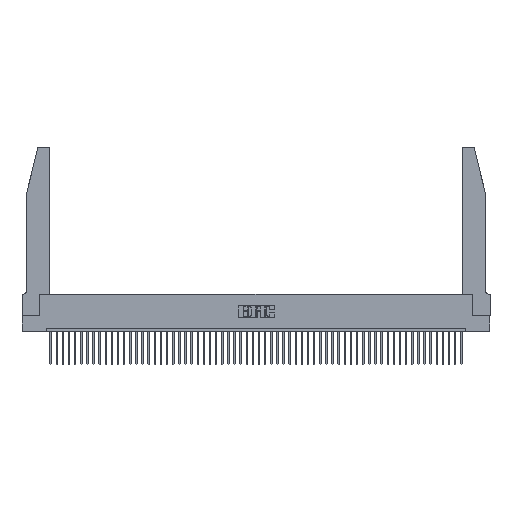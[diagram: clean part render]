
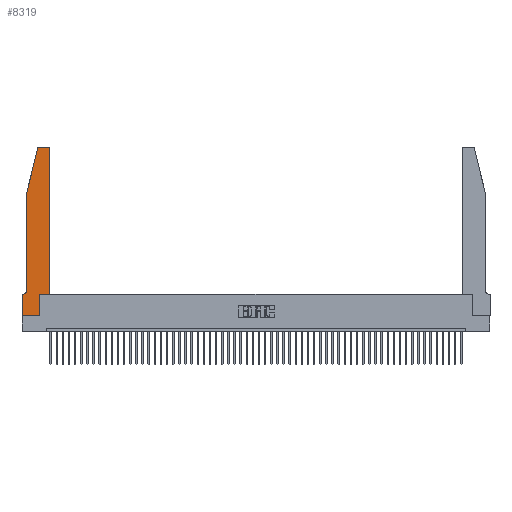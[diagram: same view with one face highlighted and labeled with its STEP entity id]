
A CAD part, top view. The second image highlights one B-rep face of the part: STEP entity #8319.
In plain terms, the highlighted planar face has unit normal (0, 0, 1).
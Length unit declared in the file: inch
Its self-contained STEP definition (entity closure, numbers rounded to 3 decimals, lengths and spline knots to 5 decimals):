
#94 = CARTESIAN_POINT ( 'NONE',  ( 0.2865, 0.35, 0.37 ) ) ;
#835 = EDGE_CURVE ( 'NONE', #48034, #19358, #24622, .T. ) ;
#1176 = DIRECTION ( 'NONE',  ( 0., -1., 0. ) ) ;
#1501 = EDGE_CURVE ( 'NONE', #41923, #16142, #8799, .T. ) ;
#1686 = EDGE_CURVE ( 'NONE', #50019, #41923, #30232, .T. ) ;
#1885 = CARTESIAN_POINT ( 'NONE',  ( 0., 0.35, 0.37 ) ) ;
#2378 = DIRECTION ( 'NONE',  ( 0., 1., 0. ) ) ;
#3093 = CARTESIAN_POINT ( 'NONE',  ( 0.0755, 2., 0.37 ) ) ;
#3177 = DIRECTION ( 'NONE',  ( 1., 0., 0. ) ) ;
#4430 = VECTOR ( 'NONE', #41938, 39.37008 ) ;
#5668 = CARTESIAN_POINT ( 'NONE',  ( 0.0755, 2., 0.37 ) ) ;
#5995 = EDGE_CURVE ( 'NONE', #42467, #19080, #8947, .T. ) ;
#6057 = DIRECTION ( 'NONE',  ( -0.239, -0.971, 0. ) ) ;
#6520 = CARTESIAN_POINT ( 'NONE',  ( 0.4505, 0.35, 0.37 ) ) ;
#6750 = EDGE_CURVE ( 'NONE', #31443, #37881, #12670, .T. ) ;
#7632 = DIRECTION ( 'NONE',  ( 1., 0., 0. ) ) ;
#7729 = CARTESIAN_POINT ( 'NONE',  ( 0., 0.35, 0.37 ) ) ;
#8019 = CARTESIAN_POINT ( 'NONE',  ( 0.284, 2.75, 0.37 ) ) ;
#8319 = ADVANCED_FACE ( 'NONE', ( #45154 ), #17947, .T. ) ;
#8657 = CARTESIAN_POINT ( 'NONE',  ( 0.0755, 0.42, 0.37 ) ) ;
#8799 = LINE ( 'NONE', #6520, #49311 ) ;
#8947 = CIRCLE ( 'NONE', #48987, 0.03 ) ;
#9010 = LINE ( 'NONE', #42286, #19774 ) ;
#9547 = CARTESIAN_POINT ( 'NONE',  ( 0., 0., 0.37 ) ) ;
#10756 = EDGE_LOOP ( 'NONE', ( #47259, #49002, #15363, #38025, #11472, #15300, #48099, #24565, #38419, #19167, #14879, #16918 ) ) ;
#11159 = CIRCLE ( 'NONE', #27255, 0.07 ) ;
#11330 = VECTOR ( 'NONE', #27096, 39.37008 ) ;
#11472 = ORIENTED_EDGE ( 'NONE', *, *, #35206, .T. ) ;
#12103 = CARTESIAN_POINT ( 'NONE',  ( 0.4205, 2.75, 0.37 ) ) ;
#12549 = CARTESIAN_POINT ( 'NONE',  ( 0.2865, 0., 0.37 ) ) ;
#12670 = LINE ( 'NONE', #19117, #39330 ) ;
#14388 = CARTESIAN_POINT ( 'NONE',  ( 0.4505, 0.35, 0.37 ) ) ;
#14649 = VERTEX_POINT ( 'NONE', #25064 ) ;
#14879 = ORIENTED_EDGE ( 'NONE', *, *, #43651, .T. ) ;
#15300 = ORIENTED_EDGE ( 'NONE', *, *, #52190, .T. ) ;
#15363 = ORIENTED_EDGE ( 'NONE', *, *, #29635, .T. ) ;
#16142 = VERTEX_POINT ( 'NONE', #29607 ) ;
#16918 = ORIENTED_EDGE ( 'NONE', *, *, #30903, .T. ) ;
#17947 = PLANE ( 'NONE',  #28448 ) ;
#19080 = VERTEX_POINT ( 'NONE', #26862 ) ;
#19117 = CARTESIAN_POINT ( 'NONE',  ( 0., 0., 0.37 ) ) ;
#19167 = ORIENTED_EDGE ( 'NONE', *, *, #1501, .T. ) ;
#19197 = CARTESIAN_POINT ( 'NONE',  ( 0.4205, 2.72, 0.37 ) ) ;
#19358 = VERTEX_POINT ( 'NONE', #8657 ) ;
#19680 = EDGE_CURVE ( 'NONE', #37881, #50019, #20442, .T. ) ;
#19774 = VECTOR ( 'NONE', #6057, 39.37008 ) ;
#19886 = CARTESIAN_POINT ( 'NONE',  ( 0., 0., 0.37 ) ) ;
#20442 = LINE ( 'NONE', #9547, #31977 ) ;
#21329 = VERTEX_POINT ( 'NONE', #31395 ) ;
#22722 = DIRECTION ( 'NONE',  ( 1., 0., 0. ) ) ;
#23263 = DIRECTION ( 'NONE',  ( 0., 0., 1. ) ) ;
#24565 = ORIENTED_EDGE ( 'NONE', *, *, #19680, .T. ) ;
#24622 = LINE ( 'NONE', #5668, #43744 ) ;
#25064 = CARTESIAN_POINT ( 'NONE',  ( 0.0055, 0.35, 0.37 ) ) ;
#26862 = CARTESIAN_POINT ( 'NONE',  ( 0.25487, 2.72718, 0.37 ) ) ;
#27096 = DIRECTION ( 'NONE',  ( 0., 1., 0. ) ) ;
#27255 = AXIS2_PLACEMENT_3D ( 'NONE', #46239, #30101, #39530 ) ;
#27636 = CARTESIAN_POINT ( 'NONE',  ( 0.2865, 0.35, 0.37 ) ) ;
#27984 = DIRECTION ( 'NONE',  ( 1., 0., 0. ) ) ;
#28448 = AXIS2_PLACEMENT_3D ( 'NONE', #1885, #46703, #22722 ) ;
#29607 = CARTESIAN_POINT ( 'NONE',  ( 0.4505, 0.35, 0.37 ) ) ;
#29635 = EDGE_CURVE ( 'NONE', #19080, #48034, #9010, .T. ) ;
#29900 = CARTESIAN_POINT ( 'NONE',  ( 0.2605, 2.75, 0.37 ) ) ;
#30040 = VECTOR ( 'NONE', #2378, 39.37008 ) ;
#30101 = DIRECTION ( 'NONE',  ( 0., 0., -1. ) ) ;
#30232 = LINE ( 'NONE', #27636, #11330 ) ;
#30903 = EDGE_CURVE ( 'NONE', #21329, #51776, #38747, .T. ) ;
#31395 = CARTESIAN_POINT ( 'NONE',  ( 0.4505, 2.72, 0.37 ) ) ;
#31443 = VERTEX_POINT ( 'NONE', #7729 ) ;
#31562 = EDGE_CURVE ( 'NONE', #51776, #42467, #38622, .T. ) ;
#31977 = VECTOR ( 'NONE', #49711, 39.37008 ) ;
#32957 = DIRECTION ( 'NONE',  ( 0., 0., 1. ) ) ;
#35206 = EDGE_CURVE ( 'NONE', #19358, #14649, #11159, .T. ) ;
#36629 = AXIS2_PLACEMENT_3D ( 'NONE', #19197, #23263, #3177 ) ;
#36683 = CARTESIAN_POINT ( 'NONE',  ( 0.284, 2.72, 0.37 ) ) ;
#36731 = LINE ( 'NONE', #51927, #47601 ) ;
#37881 = VERTEX_POINT ( 'NONE', #19886 ) ;
#38025 = ORIENTED_EDGE ( 'NONE', *, *, #835, .T. ) ;
#38419 = ORIENTED_EDGE ( 'NONE', *, *, #1686, .T. ) ;
#38622 = LINE ( 'NONE', #29900, #4430 ) ;
#38747 = CIRCLE ( 'NONE', #36629, 0.03 ) ;
#39133 = DIRECTION ( 'NONE',  ( -1., 0., 0. ) ) ;
#39330 = VECTOR ( 'NONE', #47888, 39.37008 ) ;
#39530 = DIRECTION ( 'NONE',  ( -1., 0., 0. ) ) ;
#41923 = VERTEX_POINT ( 'NONE', #94 ) ;
#41938 = DIRECTION ( 'NONE',  ( -1., 0., 0. ) ) ;
#42286 = CARTESIAN_POINT ( 'NONE',  ( 0.0755, 2., 0.37 ) ) ;
#42467 = VERTEX_POINT ( 'NONE', #8019 ) ;
#43459 = LINE ( 'NONE', #14388, #30040 ) ;
#43651 = EDGE_CURVE ( 'NONE', #16142, #21329, #43459, .T. ) ;
#43744 = VECTOR ( 'NONE', #1176, 39.37008 ) ;
#45154 = FACE_OUTER_BOUND ( 'NONE', #10756, .T. ) ;
#46239 = CARTESIAN_POINT ( 'NONE',  ( 0.0055, 0.42, 0.37 ) ) ;
#46703 = DIRECTION ( 'NONE',  ( 0., 0., 1. ) ) ;
#47259 = ORIENTED_EDGE ( 'NONE', *, *, #31562, .T. ) ;
#47601 = VECTOR ( 'NONE', #39133, 39.37008 ) ;
#47888 = DIRECTION ( 'NONE',  ( 0., -1., 0. ) ) ;
#48034 = VERTEX_POINT ( 'NONE', #3093 ) ;
#48099 = ORIENTED_EDGE ( 'NONE', *, *, #6750, .T. ) ;
#48987 = AXIS2_PLACEMENT_3D ( 'NONE', #36683, #32957, #27984 ) ;
#49002 = ORIENTED_EDGE ( 'NONE', *, *, #5995, .T. ) ;
#49311 = VECTOR ( 'NONE', #7632, 39.37008 ) ;
#49711 = DIRECTION ( 'NONE',  ( 1., 0., 0. ) ) ;
#50019 = VERTEX_POINT ( 'NONE', #12549 ) ;
#51776 = VERTEX_POINT ( 'NONE', #12103 ) ;
#51927 = CARTESIAN_POINT ( 'NONE',  ( 0.0755, 0.35, 0.37 ) ) ;
#52190 = EDGE_CURVE ( 'NONE', #14649, #31443, #36731, .T. ) ;
